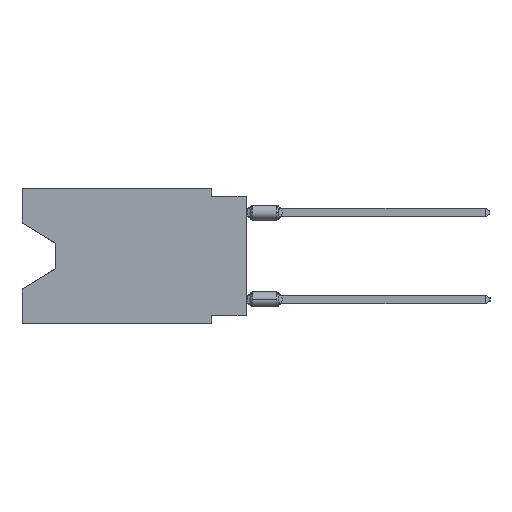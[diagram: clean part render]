
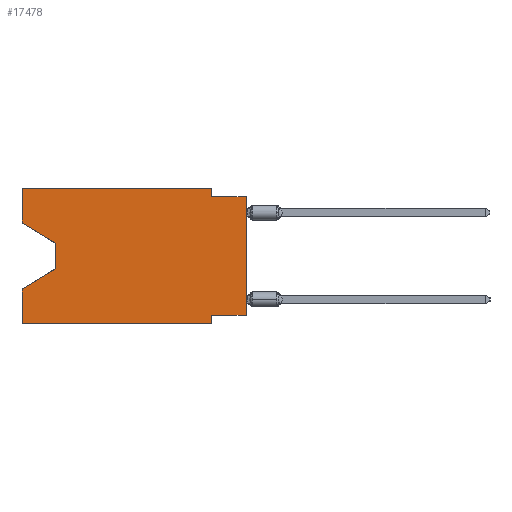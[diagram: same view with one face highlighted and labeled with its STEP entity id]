
A CAD part, left-side view. The second image highlights one B-rep face of the part: STEP entity #17478.
In plain terms, the highlighted planar face has unit normal (-1, 0, 0).
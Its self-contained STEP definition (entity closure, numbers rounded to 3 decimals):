
#452 = DIRECTION ( 'NONE',  ( 0., 0., 1. ) ) ;
#791 = ORIENTED_EDGE ( 'NONE', *, *, #3338, .F. ) ;
#1678 = VECTOR ( 'NONE', #26446, 1000. ) ;
#1865 = EDGE_CURVE ( 'NONE', #28311, #53583, #36699, .T. ) ;
#1962 = CARTESIAN_POINT ( 'NONE',  ( 0., 16.383, 0. ) ) ;
#2073 = EDGE_CURVE ( 'NONE', #38539, #21781, #7156, .T. ) ;
#3005 = CARTESIAN_POINT ( 'NONE',  ( 0., 2.54, -9.271 ) ) ;
#3338 = EDGE_CURVE ( 'NONE', #51951, #38539, #42334, .T. ) ;
#3399 = VECTOR ( 'NONE', #12630, 1000. ) ;
#3470 = LINE ( 'NONE', #11672, #36368 ) ;
#3838 = CARTESIAN_POINT ( 'NONE',  ( 0., 16.383, 0. ) ) ;
#4040 = LINE ( 'NONE', #48501, #44156 ) ;
#6174 = ORIENTED_EDGE ( 'NONE', *, *, #25624, .T. ) ;
#6436 = CARTESIAN_POINT ( 'NONE',  ( 0., 2.54, 0. ) ) ;
#6639 = CARTESIAN_POINT ( 'NONE',  ( 0., 0., -9.271 ) ) ;
#7156 = LINE ( 'NONE', #28512, #31801 ) ;
#7581 = EDGE_CURVE ( 'NONE', #55658, #51951, #25503, .T. ) ;
#8324 = LINE ( 'NONE', #48958, #1678 ) ;
#8523 = CARTESIAN_POINT ( 'NONE',  ( 0., 2.54, -9.906 ) ) ;
#9041 = VERTEX_POINT ( 'NONE', #9694 ) ;
#9228 = EDGE_CURVE ( 'NONE', #21781, #13334, #34809, .T. ) ;
#9694 = CARTESIAN_POINT ( 'NONE',  ( 0., 0., -9.271 ) ) ;
#10490 = CARTESIAN_POINT ( 'NONE',  ( 0., 16.383, -2.546 ) ) ;
#11672 = CARTESIAN_POINT ( 'NONE',  ( 0., 2.54, -9.906 ) ) ;
#12630 = DIRECTION ( 'NONE',  ( 0., 0., 1. ) ) ;
#13334 = VERTEX_POINT ( 'NONE', #40505 ) ;
#14407 = EDGE_CURVE ( 'NONE', #9041, #42490, #51973, .T. ) ;
#15864 = VECTOR ( 'NONE', #452, 1000. ) ;
#16772 = CARTESIAN_POINT ( 'NONE',  ( 0., 0., 0. ) ) ;
#17478 = ADVANCED_FACE ( 'NONE', ( #26647 ), #26077, .F. ) ;
#17537 = VERTEX_POINT ( 'NONE', #8523 ) ;
#17759 = ORIENTED_EDGE ( 'NONE', *, *, #7581, .F. ) ;
#17825 = CARTESIAN_POINT ( 'NONE',  ( 0., 16.383, 0. ) ) ;
#18405 = ORIENTED_EDGE ( 'NONE', *, *, #14407, .F. ) ;
#20757 = VECTOR ( 'NONE', #42906, 1000. ) ;
#20823 = DIRECTION ( 'NONE',  ( 0., 0.855, -0.519 ) ) ;
#21165 = DIRECTION ( 'NONE',  ( 0., 0., 1. ) ) ;
#21781 = VERTEX_POINT ( 'NONE', #34618 ) ;
#21886 = DIRECTION ( 'NONE',  ( 0., -1., 0. ) ) ;
#22114 = ORIENTED_EDGE ( 'NONE', *, *, #56252, .T. ) ;
#23518 = CARTESIAN_POINT ( 'NONE',  ( 0., 16.383, 0. ) ) ;
#23635 = LINE ( 'NONE', #10490, #48073 ) ;
#23794 = EDGE_CURVE ( 'NONE', #42490, #17537, #3470, .T. ) ;
#24619 = CARTESIAN_POINT ( 'NONE',  ( 0., 13.97, -5.893 ) ) ;
#24836 = VECTOR ( 'NONE', #52654, 1000. ) ;
#25074 = ORIENTED_EDGE ( 'NONE', *, *, #36303, .T. ) ;
#25503 = LINE ( 'NONE', #38968, #3399 ) ;
#25624 = EDGE_CURVE ( 'NONE', #28311, #17537, #4040, .T. ) ;
#25702 = DIRECTION ( 'NONE',  ( 0., 0., -1. ) ) ;
#26077 = PLANE ( 'NONE',  #50945 ) ;
#26446 = DIRECTION ( 'NONE',  ( 0., 0., -1. ) ) ;
#26647 = FACE_OUTER_BOUND ( 'NONE', #34397, .T. ) ;
#28311 = VERTEX_POINT ( 'NONE', #39177 ) ;
#28512 = CARTESIAN_POINT ( 'NONE',  ( 0., 2.54, 0. ) ) ;
#28798 = CARTESIAN_POINT ( 'NONE',  ( 0., 16.383, -2.546 ) ) ;
#29087 = DIRECTION ( 'NONE',  ( 0., 0., -1. ) ) ;
#29595 = LINE ( 'NONE', #24619, #35856 ) ;
#29837 = EDGE_CURVE ( 'NONE', #55658, #51314, #23635, .T. ) ;
#30132 = VECTOR ( 'NONE', #36774, 1000. ) ;
#31083 = LINE ( 'NONE', #16772, #51383 ) ;
#31801 = VECTOR ( 'NONE', #29087, 1000. ) ;
#32624 = ORIENTED_EDGE ( 'NONE', *, *, #9228, .F. ) ;
#34397 = EDGE_LOOP ( 'NONE', ( #42483, #38682, #22114, #50034, #6174, #52165, #18405, #25074, #32624, #39232, #791, #17759 ) ) ;
#34618 = CARTESIAN_POINT ( 'NONE',  ( 0., 2.54, -0.635 ) ) ;
#34809 = LINE ( 'NONE', #43005, #24836 ) ;
#35711 = DIRECTION ( 'NONE',  ( 0., 0., -1. ) ) ;
#35856 = VECTOR ( 'NONE', #20823, 1000. ) ;
#36303 = EDGE_CURVE ( 'NONE', #9041, #13334, #31083, .T. ) ;
#36368 = VECTOR ( 'NONE', #25702, 1000. ) ;
#36699 = LINE ( 'NONE', #23518, #15864 ) ;
#36774 = DIRECTION ( 'NONE',  ( 0., -1., 0. ) ) ;
#37390 = DIRECTION ( 'NONE',  ( 0., -0.855, -0.519 ) ) ;
#38539 = VERTEX_POINT ( 'NONE', #6436 ) ;
#38682 = ORIENTED_EDGE ( 'NONE', *, *, #39657, .T. ) ;
#38968 = CARTESIAN_POINT ( 'NONE',  ( 0., 16.383, 0. ) ) ;
#39177 = CARTESIAN_POINT ( 'NONE',  ( 0., 16.383, -9.906 ) ) ;
#39232 = ORIENTED_EDGE ( 'NONE', *, *, #2073, .F. ) ;
#39657 = EDGE_CURVE ( 'NONE', #51314, #44068, #8324, .T. ) ;
#40505 = CARTESIAN_POINT ( 'NONE',  ( 0., 0., -0.635 ) ) ;
#42334 = LINE ( 'NONE', #1962, #30132 ) ;
#42483 = ORIENTED_EDGE ( 'NONE', *, *, #29837, .T. ) ;
#42490 = VERTEX_POINT ( 'NONE', #3005 ) ;
#42906 = DIRECTION ( 'NONE',  ( 0., 1., 0. ) ) ;
#43005 = CARTESIAN_POINT ( 'NONE',  ( 0., 0., -0.635 ) ) ;
#43023 = CARTESIAN_POINT ( 'NONE',  ( 0., 13.97, -5.893 ) ) ;
#44068 = VERTEX_POINT ( 'NONE', #43023 ) ;
#44156 = VECTOR ( 'NONE', #21886, 1000. ) ;
#48073 = VECTOR ( 'NONE', #37390, 1000. ) ;
#48501 = CARTESIAN_POINT ( 'NONE',  ( 0., 16.383, -9.906 ) ) ;
#48589 = DIRECTION ( 'NONE',  ( 1., 0., 0. ) ) ;
#48958 = CARTESIAN_POINT ( 'NONE',  ( 0., 13.97, -4.013 ) ) ;
#50034 = ORIENTED_EDGE ( 'NONE', *, *, #1865, .F. ) ;
#50945 = AXIS2_PLACEMENT_3D ( 'NONE', #3838, #48589, #35711 ) ;
#51314 = VERTEX_POINT ( 'NONE', #55140 ) ;
#51383 = VECTOR ( 'NONE', #21165, 1000. ) ;
#51951 = VERTEX_POINT ( 'NONE', #17825 ) ;
#51973 = LINE ( 'NONE', #6639, #20757 ) ;
#52165 = ORIENTED_EDGE ( 'NONE', *, *, #23794, .F. ) ;
#52654 = DIRECTION ( 'NONE',  ( 0., -1., 0. ) ) ;
#53583 = VERTEX_POINT ( 'NONE', #55848 ) ;
#55140 = CARTESIAN_POINT ( 'NONE',  ( 0., 13.97, -4.013 ) ) ;
#55658 = VERTEX_POINT ( 'NONE', #28798 ) ;
#55848 = CARTESIAN_POINT ( 'NONE',  ( 0., 16.383, -7.36 ) ) ;
#56252 = EDGE_CURVE ( 'NONE', #44068, #53583, #29595, .T. ) ;
